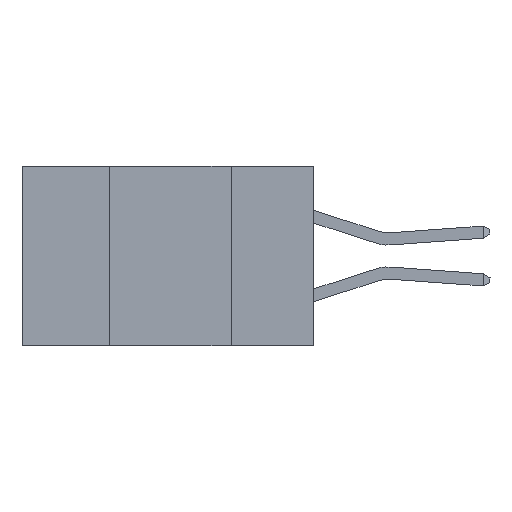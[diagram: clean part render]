
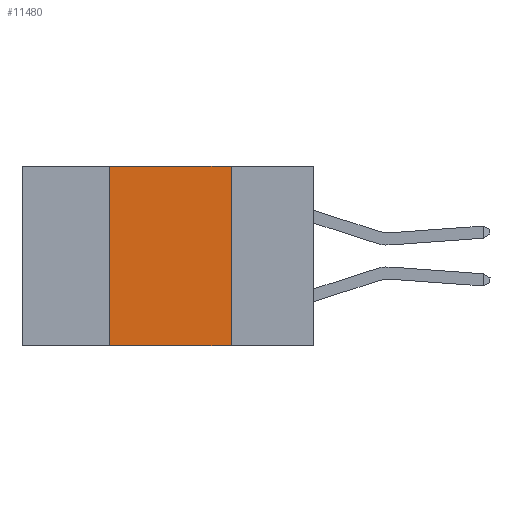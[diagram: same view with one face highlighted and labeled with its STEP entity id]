
A CAD part, left-side view. The second image highlights one B-rep face of the part: STEP entity #11480.
In plain terms, the highlighted planar face has unit normal (-1, 0, 0).
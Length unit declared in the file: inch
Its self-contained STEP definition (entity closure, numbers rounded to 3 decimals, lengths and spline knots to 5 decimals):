
#92 = EDGE_LOOP ( 'NONE', ( #1542, #395, #1752, #9836 ) ) ;
#197 = VECTOR ( 'NONE', #3602, 39.37008 ) ;
#395 = ORIENTED_EDGE ( 'NONE', *, *, #2323, .F. ) ;
#415 = CARTESIAN_POINT ( 'NONE',  ( 0., 0.17, -0.37 ) ) ;
#1333 = VECTOR ( 'NONE', #6242, 39.37008 ) ;
#1542 = ORIENTED_EDGE ( 'NONE', *, *, #2908, .F. ) ;
#1637 = PLANE ( 'NONE',  #5221 ) ;
#1752 = ORIENTED_EDGE ( 'NONE', *, *, #3235, .F. ) ;
#2323 = EDGE_CURVE ( 'NONE', #3752, #6618, #2986, .T. ) ;
#2649 = VECTOR ( 'NONE', #3315, 39.37008 ) ;
#2908 = EDGE_CURVE ( 'NONE', #6618, #11331, #12134, .T. ) ;
#2986 = LINE ( 'NONE', #7452, #2649 ) ;
#3187 = EDGE_CURVE ( 'NONE', #5588, #11331, #8496, .T. ) ;
#3235 = EDGE_CURVE ( 'NONE', #5588, #3752, #5736, .T. ) ;
#3315 = DIRECTION ( 'NONE',  ( 0., -1., 0. ) ) ;
#3602 = DIRECTION ( 'NONE',  ( 0., 0., -1. ) ) ;
#3697 = DIRECTION ( 'NONE',  ( 0., 0., -1. ) ) ;
#3752 = VERTEX_POINT ( 'NONE', #12887 ) ;
#5221 = AXIS2_PLACEMENT_3D ( 'NONE', #13181, #9022, #3697 ) ;
#5588 = VERTEX_POINT ( 'NONE', #7108 ) ;
#5736 = LINE ( 'NONE', #9082, #6710 ) ;
#5991 = DIRECTION ( 'NONE',  ( 0., 0., 1. ) ) ;
#6242 = DIRECTION ( 'NONE',  ( 0., -1., 0. ) ) ;
#6618 = VERTEX_POINT ( 'NONE', #8247 ) ;
#6710 = VECTOR ( 'NONE', #5991, 39.37008 ) ;
#7108 = CARTESIAN_POINT ( 'NONE',  ( 0., 0.42, -0.37 ) ) ;
#7452 = CARTESIAN_POINT ( 'NONE',  ( 0., 0.6, 0. ) ) ;
#8247 = CARTESIAN_POINT ( 'NONE',  ( 0., 0.17, 0. ) ) ;
#8266 = FACE_OUTER_BOUND ( 'NONE', #92, .T. ) ;
#8496 = LINE ( 'NONE', #11446, #1333 ) ;
#9022 = DIRECTION ( 'NONE',  ( 1., 0., 0. ) ) ;
#9082 = CARTESIAN_POINT ( 'NONE',  ( 0., 0.42, 0. ) ) ;
#9836 = ORIENTED_EDGE ( 'NONE', *, *, #3187, .T. ) ;
#10846 = CARTESIAN_POINT ( 'NONE',  ( 0., 0.17, 0. ) ) ;
#11331 = VERTEX_POINT ( 'NONE', #415 ) ;
#11446 = CARTESIAN_POINT ( 'NONE',  ( 0., 0.6, -0.37 ) ) ;
#11480 = ADVANCED_FACE ( 'NONE', ( #8266 ), #1637, .F. ) ;
#12134 = LINE ( 'NONE', #10846, #197 ) ;
#12887 = CARTESIAN_POINT ( 'NONE',  ( 0., 0.42, 0. ) ) ;
#13181 = CARTESIAN_POINT ( 'NONE',  ( 0., 0.6, 0. ) ) ;
